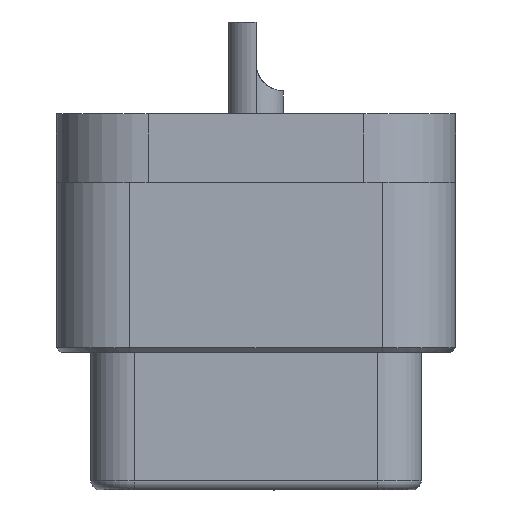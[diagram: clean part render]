
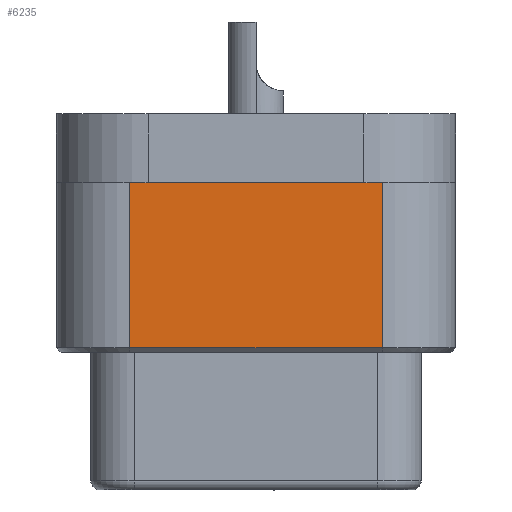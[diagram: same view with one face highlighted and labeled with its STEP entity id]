
A CAD part, left-side view. The second image highlights one B-rep face of the part: STEP entity #6235.
In plain terms, the highlighted planar face has unit normal (-1, 0, 0).
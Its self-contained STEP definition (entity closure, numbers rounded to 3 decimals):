
#142 = FACE_OUTER_BOUND ( 'NONE', #2966, .T. ) ;
#789 = ORIENTED_EDGE ( 'NONE', *, *, #5342, .T. ) ;
#797 = LINE ( 'NONE', #3264, #6818 ) ;
#1316 = CARTESIAN_POINT ( 'NONE',  ( -10.6, 97.25, 16.6 ) ) ;
#1358 = CARTESIAN_POINT ( 'NONE',  ( -10.6, 102.75, 20.2 ) ) ;
#1996 = DIRECTION ( 'NONE',  ( 0., 1., 0. ) ) ;
#2074 = DIRECTION ( 'NONE',  ( 0., 0., 1. ) ) ;
#2208 = ORIENTED_EDGE ( 'NONE', *, *, #3932, .F. ) ;
#2286 = CARTESIAN_POINT ( 'NONE',  ( -10.6, 102.75, 16.6 ) ) ;
#2608 = PLANE ( 'NONE',  #5465 ) ;
#2707 = VECTOR ( 'NONE', #2074, 1000. ) ;
#2966 = EDGE_LOOP ( 'NONE', ( #7080, #5628, #2208, #789 ) ) ;
#3030 = VECTOR ( 'NONE', #3817, 1000. ) ;
#3222 = CARTESIAN_POINT ( 'NONE',  ( -10.6, 102.75, 16.6 ) ) ;
#3264 = CARTESIAN_POINT ( 'NONE',  ( -10.6, 102.75, 20.2 ) ) ;
#3817 = DIRECTION ( 'NONE',  ( 0., -1., 0. ) ) ;
#3841 = CARTESIAN_POINT ( 'NONE',  ( -10.6, 97.25, 20.2 ) ) ;
#3932 = EDGE_CURVE ( 'NONE', #6427, #5551, #6867, .T. ) ;
#4187 = EDGE_CURVE ( 'NONE', #7747, #5303, #7782, .T. ) ;
#4728 = DIRECTION ( 'NONE',  ( 0., -1., 0. ) ) ;
#5052 = CARTESIAN_POINT ( 'NONE',  ( -10.6, 100., 18.4 ) ) ;
#5126 = LINE ( 'NONE', #7568, #2707 ) ;
#5303 = VERTEX_POINT ( 'NONE', #1316 ) ;
#5342 = EDGE_CURVE ( 'NONE', #6427, #7747, #797, .T. ) ;
#5465 = AXIS2_PLACEMENT_3D ( 'NONE', #5052, #7498, #1996 ) ;
#5551 = VERTEX_POINT ( 'NONE', #3841 ) ;
#5588 = VECTOR ( 'NONE', #4728, 1000. ) ;
#5628 = ORIENTED_EDGE ( 'NONE', *, *, #6772, .T. ) ;
#5708 = DIRECTION ( 'NONE',  ( 0., 0., -1. ) ) ;
#5879 = CARTESIAN_POINT ( 'NONE',  ( -10.6, 102.75, 20.2 ) ) ;
#6235 = ADVANCED_FACE ( 'NONE', ( #142 ), #2608, .F. ) ;
#6427 = VERTEX_POINT ( 'NONE', #5879 ) ;
#6772 = EDGE_CURVE ( 'NONE', #5303, #5551, #5126, .T. ) ;
#6818 = VECTOR ( 'NONE', #5708, 1000. ) ;
#6867 = LINE ( 'NONE', #1358, #3030 ) ;
#7080 = ORIENTED_EDGE ( 'NONE', *, *, #4187, .T. ) ;
#7498 = DIRECTION ( 'NONE',  ( 1., 0., 0. ) ) ;
#7568 = CARTESIAN_POINT ( 'NONE',  ( -10.6, 97.25, 16.6 ) ) ;
#7747 = VERTEX_POINT ( 'NONE', #3222 ) ;
#7782 = LINE ( 'NONE', #2286, #5588 ) ;
